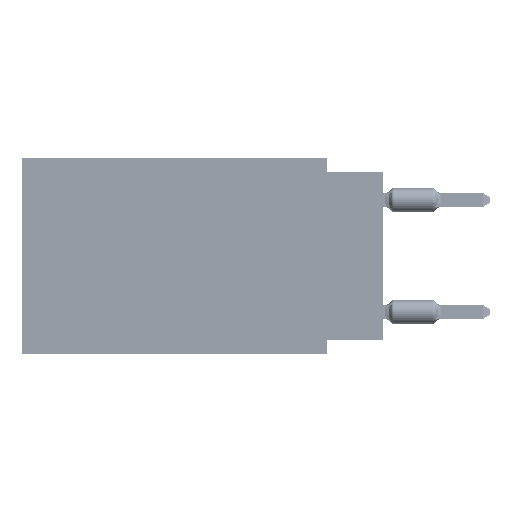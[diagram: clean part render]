
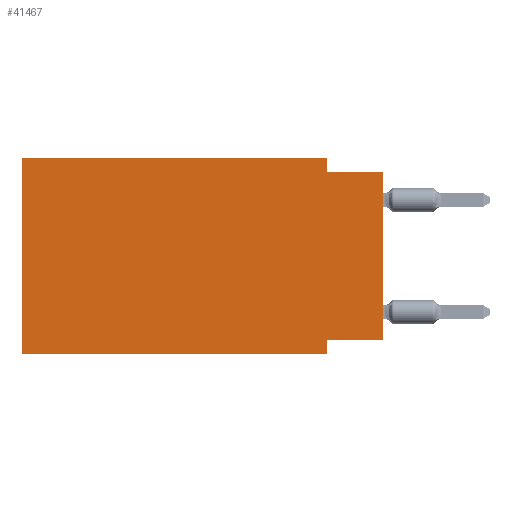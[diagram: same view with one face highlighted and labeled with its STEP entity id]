
A CAD part, left-side view. The second image highlights one B-rep face of the part: STEP entity #41467.
In plain terms, the highlighted planar face has unit normal (-1, 0, 0).
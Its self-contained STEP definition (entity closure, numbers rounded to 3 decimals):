
#618 = CARTESIAN_POINT ( 'NONE',  ( 0., 0., -8.255 ) ) ;
#4068 = VECTOR ( 'NONE', #67988, 1000. ) ;
#8757 = ORIENTED_EDGE ( 'NONE', *, *, #64225, .F. ) ;
#9303 = LINE ( 'NONE', #41638, #4068 ) ;
#9348 = DIRECTION ( 'NONE',  ( 0., -1., 0. ) ) ;
#9368 = CARTESIAN_POINT ( 'NONE',  ( 0., 2.54, -8.89 ) ) ;
#9404 = LINE ( 'NONE', #10448, #65191 ) ;
#9705 = DIRECTION ( 'NONE',  ( 0., 0., -1. ) ) ;
#10448 = CARTESIAN_POINT ( 'NONE',  ( 0., 2.54, 0. ) ) ;
#11874 = AXIS2_PLACEMENT_3D ( 'NONE', #31862, #69436, #9705 ) ;
#12642 = LINE ( 'NONE', #43932, #59956 ) ;
#13116 = CARTESIAN_POINT ( 'NONE',  ( 0., 0., -0.635 ) ) ;
#13670 = VECTOR ( 'NONE', #68712, 1000. ) ;
#13911 = LINE ( 'NONE', #14259, #39746 ) ;
#14259 = CARTESIAN_POINT ( 'NONE',  ( 0., 16.383, -8.89 ) ) ;
#15367 = VECTOR ( 'NONE', #47899, 1000. ) ;
#15370 = CARTESIAN_POINT ( 'NONE',  ( 0., 0., -0.635 ) ) ;
#21326 = DIRECTION ( 'NONE',  ( 0., 0., -1. ) ) ;
#21555 = CARTESIAN_POINT ( 'NONE',  ( 0., 0., 0. ) ) ;
#22064 = DIRECTION ( 'NONE',  ( 0., 1., 0. ) ) ;
#22194 = LINE ( 'NONE', #43988, #13670 ) ;
#23461 = EDGE_CURVE ( 'NONE', #48291, #56643, #12642, .T. ) ;
#24978 = EDGE_CURVE ( 'NONE', #35971, #48087, #48773, .T. ) ;
#26901 = VERTEX_POINT ( 'NONE', #45077 ) ;
#28266 = DIRECTION ( 'NONE',  ( 0., -1., 0. ) ) ;
#28974 = EDGE_CURVE ( 'NONE', #56643, #26901, #9404, .T. ) ;
#29489 = ORIENTED_EDGE ( 'NONE', *, *, #23461, .F. ) ;
#29965 = EDGE_CURVE ( 'NONE', #48087, #45265, #22194, .T. ) ;
#31862 = CARTESIAN_POINT ( 'NONE',  ( 0., 16.383, 0. ) ) ;
#35685 = EDGE_LOOP ( 'NONE', ( #38414, #8757, #64936, #29489, #56757, #50669, #60186, #53971 ) ) ;
#35971 = VERTEX_POINT ( 'NONE', #40553 ) ;
#37764 = EDGE_CURVE ( 'NONE', #52228, #45265, #13911, .T. ) ;
#38414 = ORIENTED_EDGE ( 'NONE', *, *, #45334, .T. ) ;
#39746 = VECTOR ( 'NONE', #9348, 1000. ) ;
#40553 = CARTESIAN_POINT ( 'NONE',  ( 0., 0., -8.255 ) ) ;
#41043 = VECTOR ( 'NONE', #22064, 1000. ) ;
#41203 = CARTESIAN_POINT ( 'NONE',  ( 0., 2.54, -8.255 ) ) ;
#41268 = VECTOR ( 'NONE', #28266, 1000. ) ;
#41467 = ADVANCED_FACE ( 'NONE', ( #57833 ), #58174, .F. ) ;
#41638 = CARTESIAN_POINT ( 'NONE',  ( 0., 16.383, 0. ) ) ;
#43608 = CARTESIAN_POINT ( 'NONE',  ( 0., 16.383, -8.89 ) ) ;
#43932 = CARTESIAN_POINT ( 'NONE',  ( 0., 16.383, 0. ) ) ;
#43988 = CARTESIAN_POINT ( 'NONE',  ( 0., 2.54, -8.89 ) ) ;
#44161 = EDGE_CURVE ( 'NONE', #52228, #48291, #9303, .T. ) ;
#45077 = CARTESIAN_POINT ( 'NONE',  ( 0., 2.54, -0.635 ) ) ;
#45265 = VERTEX_POINT ( 'NONE', #9368 ) ;
#45334 = EDGE_CURVE ( 'NONE', #35971, #63545, #48243, .T. ) ;
#47899 = DIRECTION ( 'NONE',  ( 0., 0., 1. ) ) ;
#48087 = VERTEX_POINT ( 'NONE', #41203 ) ;
#48243 = LINE ( 'NONE', #21555, #15367 ) ;
#48291 = VERTEX_POINT ( 'NONE', #50284 ) ;
#48773 = LINE ( 'NONE', #618, #41043 ) ;
#50284 = CARTESIAN_POINT ( 'NONE',  ( 0., 16.383, 0. ) ) ;
#50669 = ORIENTED_EDGE ( 'NONE', *, *, #37764, .T. ) ;
#52228 = VERTEX_POINT ( 'NONE', #43608 ) ;
#53971 = ORIENTED_EDGE ( 'NONE', *, *, #24978, .F. ) ;
#56643 = VERTEX_POINT ( 'NONE', #67488 ) ;
#56757 = ORIENTED_EDGE ( 'NONE', *, *, #44161, .F. ) ;
#57833 = FACE_OUTER_BOUND ( 'NONE', #35685, .T. ) ;
#58174 = PLANE ( 'NONE',  #11874 ) ;
#59956 = VECTOR ( 'NONE', #65359, 1000. ) ;
#60186 = ORIENTED_EDGE ( 'NONE', *, *, #29965, .F. ) ;
#60922 = LINE ( 'NONE', #13116, #41268 ) ;
#63545 = VERTEX_POINT ( 'NONE', #15370 ) ;
#64225 = EDGE_CURVE ( 'NONE', #26901, #63545, #60922, .T. ) ;
#64936 = ORIENTED_EDGE ( 'NONE', *, *, #28974, .F. ) ;
#65191 = VECTOR ( 'NONE', #21326, 1000. ) ;
#65359 = DIRECTION ( 'NONE',  ( 0., -1., 0. ) ) ;
#67488 = CARTESIAN_POINT ( 'NONE',  ( 0., 2.54, 0. ) ) ;
#67988 = DIRECTION ( 'NONE',  ( 0., 0., 1. ) ) ;
#68712 = DIRECTION ( 'NONE',  ( 0., 0., -1. ) ) ;
#69436 = DIRECTION ( 'NONE',  ( 1., 0., 0. ) ) ;
